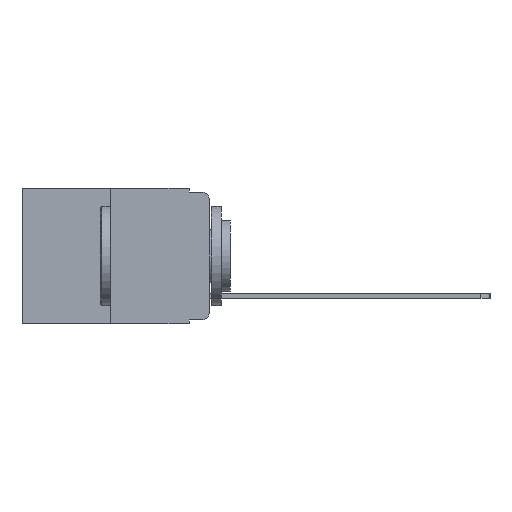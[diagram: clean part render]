
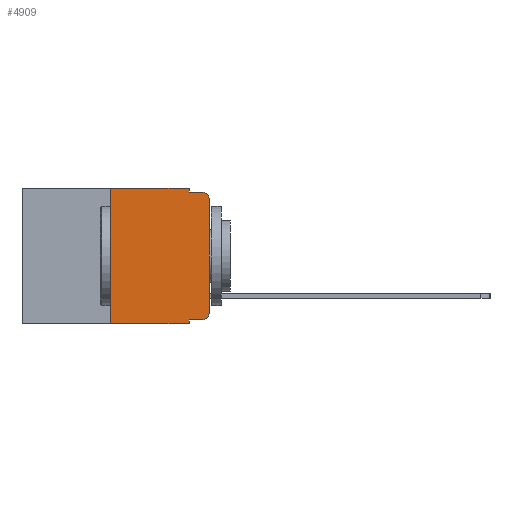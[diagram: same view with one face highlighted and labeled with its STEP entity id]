
A CAD part, left-side view. The second image highlights one B-rep face of the part: STEP entity #4909.
In plain terms, the highlighted planar face has unit normal (-1, 0, 0).
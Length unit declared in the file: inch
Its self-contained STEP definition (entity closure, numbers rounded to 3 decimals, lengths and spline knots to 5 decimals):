
#40 = DIRECTION ( 'NONE',  ( 0., 0., -1. ) ) ;
#192 = CARTESIAN_POINT ( 'NONE',  ( 0., 0., -0.03 ) ) ;
#355 = DIRECTION ( 'NONE',  ( 0., 0., 1. ) ) ;
#677 = ORIENTED_EDGE ( 'NONE', *, *, #5228, .T. ) ;
#750 = DIRECTION ( 'NONE',  ( 0., 0., -1. ) ) ;
#811 = CARTESIAN_POINT ( 'NONE',  ( 0., 0., 0. ) ) ;
#826 = DIRECTION ( 'NONE',  ( 0., 0., 1. ) ) ;
#829 = CARTESIAN_POINT ( 'NONE',  ( 0., 0.051, -0.333 ) ) ;
#964 = VERTEX_POINT ( 'NONE', #4728 ) ;
#989 = DIRECTION ( 'NONE',  ( 0., -1., 0. ) ) ;
#1035 = ORIENTED_EDGE ( 'NONE', *, *, #10155, .T. ) ;
#1208 = ORIENTED_EDGE ( 'NONE', *, *, #2081, .T. ) ;
#1572 = VECTOR ( 'NONE', #8393, 39.37008 ) ;
#1772 = CARTESIAN_POINT ( 'NONE',  ( 0., 0.02, -0.313 ) ) ;
#1862 = ORIENTED_EDGE ( 'NONE', *, *, #9076, .F. ) ;
#1961 = LINE ( 'NONE', #6635, #6491 ) ;
#2081 = EDGE_CURVE ( 'NONE', #4201, #6338, #11916, .T. ) ;
#2107 = VERTEX_POINT ( 'NONE', #10715 ) ;
#2135 = LINE ( 'NONE', #11993, #6959 ) ;
#2374 = DIRECTION ( 'NONE',  ( -1., 0., 0. ) ) ;
#2689 = VERTEX_POINT ( 'NONE', #11518 ) ;
#2695 = EDGE_CURVE ( 'NONE', #2689, #964, #5629, .T. ) ;
#2777 = DIRECTION ( 'NONE',  ( 0., 0., -1. ) ) ;
#3082 = VECTOR ( 'NONE', #8406, 39.37008 ) ;
#3161 = AXIS2_PLACEMENT_3D ( 'NONE', #1772, #8454, #2777 ) ;
#3219 = VERTEX_POINT ( 'NONE', #6389 ) ;
#3627 = CARTESIAN_POINT ( 'NONE',  ( 0., 0.02, -0.03 ) ) ;
#4049 = VECTOR ( 'NONE', #989, 39.37008 ) ;
#4201 = VERTEX_POINT ( 'NONE', #6336 ) ;
#4231 = DIRECTION ( 'NONE',  ( 0., -1., 0. ) ) ;
#4398 = CARTESIAN_POINT ( 'NONE',  ( 0., 0.25, 0. ) ) ;
#4509 = LINE ( 'NONE', #11585, #11544 ) ;
#4638 = CARTESIAN_POINT ( 'NONE',  ( 0., 0.051, -0.01 ) ) ;
#4657 = DIRECTION ( 'NONE',  ( 0., -1., 0. ) ) ;
#4728 = CARTESIAN_POINT ( 'NONE',  ( 0., 0.051, 0. ) ) ;
#4753 = ORIENTED_EDGE ( 'NONE', *, *, #2695, .F. ) ;
#4909 = ADVANCED_FACE ( 'NONE', ( #5690 ), #8214, .F. ) ;
#5228 = EDGE_CURVE ( 'NONE', #2107, #8141, #6574, .T. ) ;
#5363 = ORIENTED_EDGE ( 'NONE', *, *, #5465, .F. ) ;
#5465 = EDGE_CURVE ( 'NONE', #2107, #8729, #9438, .T. ) ;
#5629 = LINE ( 'NONE', #6652, #3082 ) ;
#5690 = FACE_OUTER_BOUND ( 'NONE', #11645, .T. ) ;
#6336 = CARTESIAN_POINT ( 'NONE',  ( 0., 0., -0.313 ) ) ;
#6338 = VERTEX_POINT ( 'NONE', #192 ) ;
#6389 = CARTESIAN_POINT ( 'NONE',  ( 0., 0.02, -0.01 ) ) ;
#6491 = VECTOR ( 'NONE', #750, 39.37008 ) ;
#6574 = LINE ( 'NONE', #829, #4049 ) ;
#6635 = CARTESIAN_POINT ( 'NONE',  ( 0., 0.051, 0. ) ) ;
#6639 = VECTOR ( 'NONE', #355, 39.37008 ) ;
#6652 = CARTESIAN_POINT ( 'NONE',  ( 0., 0.473, 0. ) ) ;
#6959 = VECTOR ( 'NONE', #4657, 39.37008 ) ;
#7080 = VERTEX_POINT ( 'NONE', #4638 ) ;
#7299 = EDGE_CURVE ( 'NONE', #6338, #3219, #9550, .T. ) ;
#7947 = CARTESIAN_POINT ( 'NONE',  ( 0., 0.473, 0. ) ) ;
#8054 = CIRCLE ( 'NONE', #3161, 0.02 ) ;
#8094 = DIRECTION ( 'NONE',  ( 0., 0., -1. ) ) ;
#8141 = VERTEX_POINT ( 'NONE', #10681 ) ;
#8195 = DIRECTION ( 'NONE',  ( 1., 0., 0. ) ) ;
#8214 = PLANE ( 'NONE',  #11712 ) ;
#8247 = VERTEX_POINT ( 'NONE', #9958 ) ;
#8393 = DIRECTION ( 'NONE',  ( 0., 0., -1. ) ) ;
#8400 = EDGE_CURVE ( 'NONE', #8247, #8729, #2135, .T. ) ;
#8406 = DIRECTION ( 'NONE',  ( 0., -1., 0. ) ) ;
#8454 = DIRECTION ( 'NONE',  ( -1., 0., 0. ) ) ;
#8576 = CARTESIAN_POINT ( 'NONE',  ( 0., 0.051, 0. ) ) ;
#8729 = VERTEX_POINT ( 'NONE', #11592 ) ;
#8820 = EDGE_CURVE ( 'NONE', #8247, #2689, #9107, .T. ) ;
#9076 = EDGE_CURVE ( 'NONE', #964, #7080, #1961, .T. ) ;
#9107 = LINE ( 'NONE', #4398, #6639 ) ;
#9144 = ORIENTED_EDGE ( 'NONE', *, *, #7299, .T. ) ;
#9438 = LINE ( 'NONE', #8576, #1572 ) ;
#9550 = CIRCLE ( 'NONE', #12335, 0.02 ) ;
#9958 = CARTESIAN_POINT ( 'NONE',  ( 0., 0.25, -0.343 ) ) ;
#9964 = ORIENTED_EDGE ( 'NONE', *, *, #8820, .F. ) ;
#10155 = EDGE_CURVE ( 'NONE', #8141, #4201, #8054, .T. ) ;
#10463 = EDGE_CURVE ( 'NONE', #7080, #3219, #4509, .T. ) ;
#10681 = CARTESIAN_POINT ( 'NONE',  ( 0., 0.02, -0.333 ) ) ;
#10715 = CARTESIAN_POINT ( 'NONE',  ( 0., 0.051, -0.333 ) ) ;
#11496 = ORIENTED_EDGE ( 'NONE', *, *, #10463, .F. ) ;
#11518 = CARTESIAN_POINT ( 'NONE',  ( 0., 0.25, 0. ) ) ;
#11544 = VECTOR ( 'NONE', #4231, 39.37008 ) ;
#11585 = CARTESIAN_POINT ( 'NONE',  ( 0., 0.051, -0.01 ) ) ;
#11592 = CARTESIAN_POINT ( 'NONE',  ( 0., 0.051, -0.343 ) ) ;
#11634 = VECTOR ( 'NONE', #826, 39.37008 ) ;
#11645 = EDGE_LOOP ( 'NONE', ( #1208, #9144, #11496, #1862, #4753, #9964, #12349, #5363, #677, #1035 ) ) ;
#11712 = AXIS2_PLACEMENT_3D ( 'NONE', #7947, #8195, #8094 ) ;
#11916 = LINE ( 'NONE', #811, #11634 ) ;
#11993 = CARTESIAN_POINT ( 'NONE',  ( 0., 0.473, -0.343 ) ) ;
#12335 = AXIS2_PLACEMENT_3D ( 'NONE', #3627, #2374, #40 ) ;
#12349 = ORIENTED_EDGE ( 'NONE', *, *, #8400, .T. ) ;
